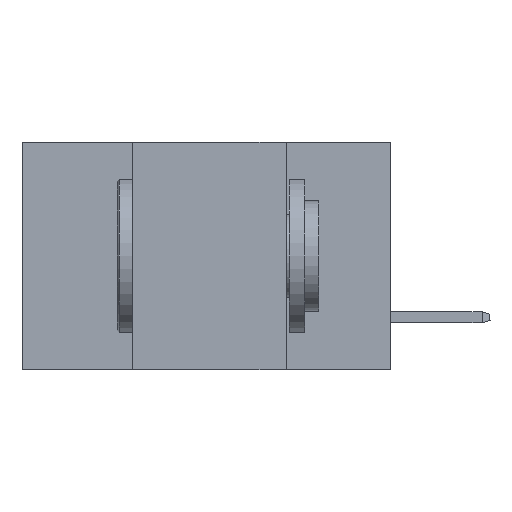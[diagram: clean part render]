
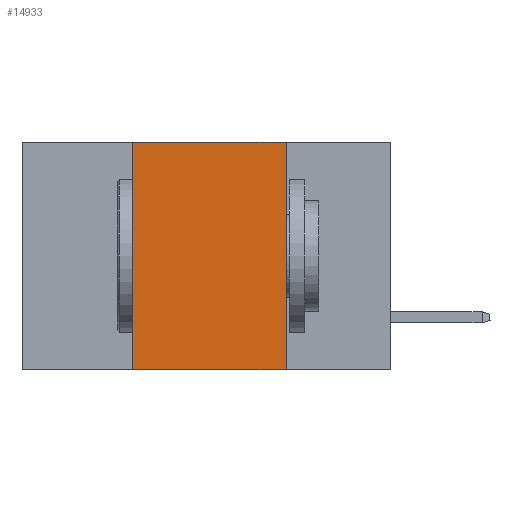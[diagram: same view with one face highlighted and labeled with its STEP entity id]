
A CAD part, left-side view. The second image highlights one B-rep face of the part: STEP entity #14933.
In plain terms, the highlighted planar face has unit normal (-1, 0, 0).
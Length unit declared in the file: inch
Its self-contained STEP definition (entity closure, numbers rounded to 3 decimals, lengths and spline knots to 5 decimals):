
#298 = VERTEX_POINT ( 'NONE', #16969 ) ;
#601 = VECTOR ( 'NONE', #12347, 39.37008 ) ;
#635 = VECTOR ( 'NONE', #19071, 39.37008 ) ;
#1015 = ORIENTED_EDGE ( 'NONE', *, *, #2092, .F. ) ;
#1194 = DIRECTION ( 'NONE',  ( 0., 0., -1. ) ) ;
#1221 = CARTESIAN_POINT ( 'NONE',  ( 0., 0.42, 0. ) ) ;
#2092 = EDGE_CURVE ( 'NONE', #16213, #298, #18628, .T. ) ;
#3007 = PLANE ( 'NONE',  #18338 ) ;
#3280 = CARTESIAN_POINT ( 'NONE',  ( 0., 0.6, 0. ) ) ;
#3294 = LINE ( 'NONE', #12033, #7055 ) ;
#3837 = ORIENTED_EDGE ( 'NONE', *, *, #8377, .F. ) ;
#4292 = VECTOR ( 'NONE', #19789, 39.37008 ) ;
#4452 = ORIENTED_EDGE ( 'NONE', *, *, #11024, .T. ) ;
#5725 = DIRECTION ( 'NONE',  ( 0., 0., -1. ) ) ;
#6847 = EDGE_CURVE ( 'NONE', #16495, #16213, #9870, .T. ) ;
#7055 = VECTOR ( 'NONE', #5725, 39.37008 ) ;
#8377 = EDGE_CURVE ( 'NONE', #298, #17173, #3294, .T. ) ;
#9104 = CARTESIAN_POINT ( 'NONE',  ( 0., 0.42, 0. ) ) ;
#9870 = LINE ( 'NONE', #1221, #601 ) ;
#10040 = CARTESIAN_POINT ( 'NONE',  ( 0., 0.6, -0.37 ) ) ;
#10472 = CARTESIAN_POINT ( 'NONE',  ( 0., 0.42, -0.37 ) ) ;
#10798 = DIRECTION ( 'NONE',  ( 1., 0., 0. ) ) ;
#11024 = EDGE_CURVE ( 'NONE', #16495, #17173, #12779, .T. ) ;
#12033 = CARTESIAN_POINT ( 'NONE',  ( 0., 0.17, 0. ) ) ;
#12347 = DIRECTION ( 'NONE',  ( 0., 0., 1. ) ) ;
#12779 = LINE ( 'NONE', #10040, #4292 ) ;
#13350 = FACE_OUTER_BOUND ( 'NONE', #13656, .T. ) ;
#13656 = EDGE_LOOP ( 'NONE', ( #3837, #1015, #18130, #4452 ) ) ;
#14933 = ADVANCED_FACE ( 'NONE', ( #13350 ), #3007, .F. ) ;
#16213 = VERTEX_POINT ( 'NONE', #9104 ) ;
#16495 = VERTEX_POINT ( 'NONE', #10472 ) ;
#16969 = CARTESIAN_POINT ( 'NONE',  ( 0., 0.17, 0. ) ) ;
#17173 = VERTEX_POINT ( 'NONE', #19105 ) ;
#18130 = ORIENTED_EDGE ( 'NONE', *, *, #6847, .F. ) ;
#18338 = AXIS2_PLACEMENT_3D ( 'NONE', #20352, #10798, #1194 ) ;
#18628 = LINE ( 'NONE', #3280, #635 ) ;
#19071 = DIRECTION ( 'NONE',  ( 0., -1., 0. ) ) ;
#19105 = CARTESIAN_POINT ( 'NONE',  ( 0., 0.17, -0.37 ) ) ;
#19789 = DIRECTION ( 'NONE',  ( 0., -1., 0. ) ) ;
#20352 = CARTESIAN_POINT ( 'NONE',  ( 0., 0.6, 0. ) ) ;
